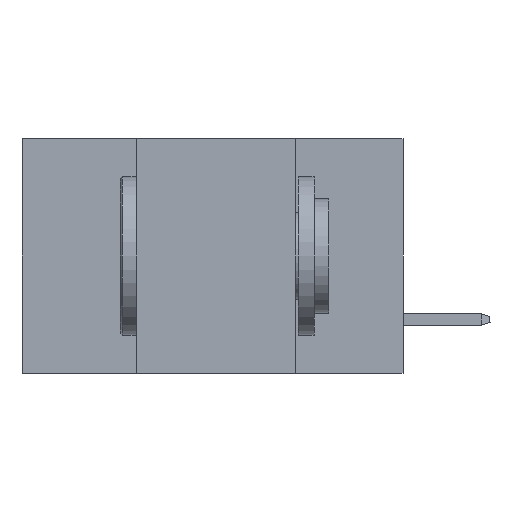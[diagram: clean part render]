
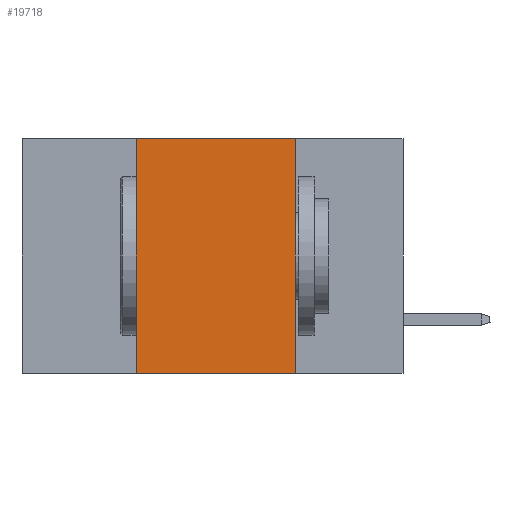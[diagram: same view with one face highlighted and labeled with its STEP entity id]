
A CAD part, left-side view. The second image highlights one B-rep face of the part: STEP entity #19718.
In plain terms, the highlighted planar face has unit normal (-1, 0, 0).
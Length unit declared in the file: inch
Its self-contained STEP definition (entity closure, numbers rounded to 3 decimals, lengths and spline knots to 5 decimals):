
#151 = PLANE ( 'NONE',  #12299 ) ;
#653 = DIRECTION ( 'NONE',  ( 1., 0., 0. ) ) ;
#1943 = VERTEX_POINT ( 'NONE', #4993 ) ;
#2240 = DIRECTION ( 'NONE',  ( 0., 0., -1. ) ) ;
#3177 = CARTESIAN_POINT ( 'NONE',  ( 0., 0.6, 0. ) ) ;
#4952 = LINE ( 'NONE', #23609, #31295 ) ;
#4993 = CARTESIAN_POINT ( 'NONE',  ( 0., 0.42, 0. ) ) ;
#6374 = ORIENTED_EDGE ( 'NONE', *, *, #27866, .F. ) ;
#6724 = CARTESIAN_POINT ( 'NONE',  ( 0., 0.17, 0. ) ) ;
#7470 = VERTEX_POINT ( 'NONE', #17801 ) ;
#8919 = LINE ( 'NONE', #19852, #24369 ) ;
#11213 = EDGE_LOOP ( 'NONE', ( #29368, #6374, #19855, #31805 ) ) ;
#12299 = AXIS2_PLACEMENT_3D ( 'NONE', #13728, #653, #29719 ) ;
#13728 = CARTESIAN_POINT ( 'NONE',  ( 0., 0.6, 0. ) ) ;
#16915 = LINE ( 'NONE', #3177, #27600 ) ;
#17801 = CARTESIAN_POINT ( 'NONE',  ( 0., 0.17, -0.37 ) ) ;
#18408 = FACE_OUTER_BOUND ( 'NONE', #11213, .T. ) ;
#19718 = ADVANCED_FACE ( 'NONE', ( #18408 ), #151, .F. ) ;
#19852 = CARTESIAN_POINT ( 'NONE',  ( 0., 0.6, -0.37 ) ) ;
#19855 = ORIENTED_EDGE ( 'NONE', *, *, #22266, .F. ) ;
#20363 = LINE ( 'NONE', #31109, #26789 ) ;
#20619 = DIRECTION ( 'NONE',  ( 0., 0., 1. ) ) ;
#20863 = EDGE_CURVE ( 'NONE', #25122, #7470, #20363, .T. ) ;
#21437 = VERTEX_POINT ( 'NONE', #31917 ) ;
#22266 = EDGE_CURVE ( 'NONE', #21437, #1943, #4952, .T. ) ;
#23609 = CARTESIAN_POINT ( 'NONE',  ( 0., 0.42, 0. ) ) ;
#24369 = VECTOR ( 'NONE', #30281, 39.37008 ) ;
#25122 = VERTEX_POINT ( 'NONE', #6724 ) ;
#26789 = VECTOR ( 'NONE', #2240, 39.37008 ) ;
#27600 = VECTOR ( 'NONE', #29612, 39.37008 ) ;
#27866 = EDGE_CURVE ( 'NONE', #1943, #25122, #16915, .T. ) ;
#29368 = ORIENTED_EDGE ( 'NONE', *, *, #20863, .F. ) ;
#29612 = DIRECTION ( 'NONE',  ( 0., -1., 0. ) ) ;
#29719 = DIRECTION ( 'NONE',  ( 0., 0., -1. ) ) ;
#30281 = DIRECTION ( 'NONE',  ( 0., -1., 0. ) ) ;
#30713 = EDGE_CURVE ( 'NONE', #21437, #7470, #8919, .T. ) ;
#31109 = CARTESIAN_POINT ( 'NONE',  ( 0., 0.17, 0. ) ) ;
#31295 = VECTOR ( 'NONE', #20619, 39.37008 ) ;
#31805 = ORIENTED_EDGE ( 'NONE', *, *, #30713, .T. ) ;
#31917 = CARTESIAN_POINT ( 'NONE',  ( 0., 0.42, -0.37 ) ) ;
